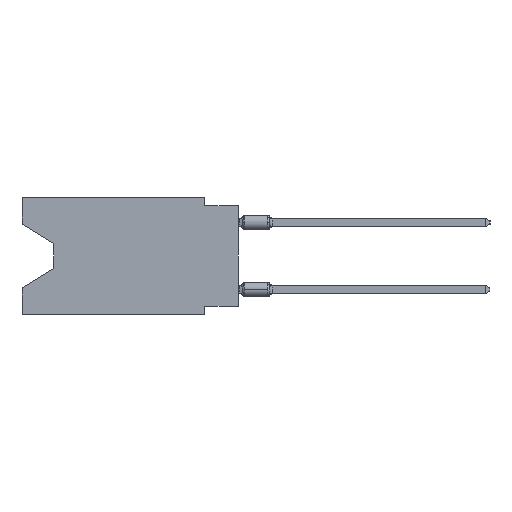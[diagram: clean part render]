
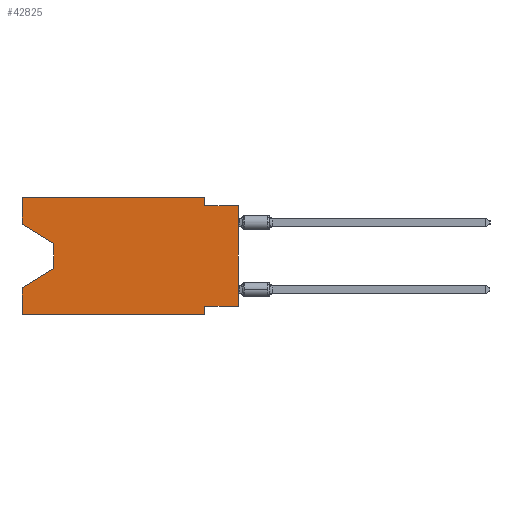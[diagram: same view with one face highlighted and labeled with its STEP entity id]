
A CAD part, left-side view. The second image highlights one B-rep face of the part: STEP entity #42825.
In plain terms, the highlighted planar face has unit normal (-1, 0, 0).
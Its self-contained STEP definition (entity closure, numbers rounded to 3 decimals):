
#413 = VERTEX_POINT ( 'NONE', #1573 ) ;
#453 = EDGE_CURVE ( 'NONE', #9264, #36588, #47007, .T. ) ;
#728 = ORIENTED_EDGE ( 'NONE', *, *, #28625, .T. ) ;
#846 = EDGE_CURVE ( 'NONE', #4577, #4938, #35246, .T. ) ;
#1457 = VERTEX_POINT ( 'NONE', #25924 ) ;
#1476 = VERTEX_POINT ( 'NONE', #22932 ) ;
#1573 = CARTESIAN_POINT ( 'NONE',  ( 0., 2.54, -0.635 ) ) ;
#1760 = EDGE_LOOP ( 'NONE', ( #43189, #728, #45736, #14791, #30633, #1821, #18890, #32439, #21754, #11471, #21118, #30006 ) ) ;
#1821 = ORIENTED_EDGE ( 'NONE', *, *, #45792, .F. ) ;
#2199 = CARTESIAN_POINT ( 'NONE',  ( 0., 0., -0.635 ) ) ;
#2579 = LINE ( 'NONE', #36806, #14096 ) ;
#3229 = LINE ( 'NONE', #21610, #23367 ) ;
#4577 = VERTEX_POINT ( 'NONE', #17387 ) ;
#4938 = VERTEX_POINT ( 'NONE', #22803 ) ;
#5269 = CARTESIAN_POINT ( 'NONE',  ( 0., 0., -0.635 ) ) ;
#7026 = VECTOR ( 'NONE', #13590, 1000. ) ;
#7044 = DIRECTION ( 'NONE',  ( 0., -0.855, -0.519 ) ) ;
#7369 = VERTEX_POINT ( 'NONE', #48970 ) ;
#7563 = VECTOR ( 'NONE', #43129, 1000. ) ;
#9264 = VERTEX_POINT ( 'NONE', #17557 ) ;
#10721 = DIRECTION ( 'NONE',  ( 0., -1., 0. ) ) ;
#11295 = EDGE_CURVE ( 'NONE', #19260, #7369, #37033, .T. ) ;
#11471 = ORIENTED_EDGE ( 'NONE', *, *, #38206, .F. ) ;
#11956 = VECTOR ( 'NONE', #24663, 1000. ) ;
#11966 = EDGE_CURVE ( 'NONE', #16822, #4938, #25248, .T. ) ;
#12874 = DIRECTION ( 'NONE',  ( 0., -1., 0. ) ) ;
#13163 = DIRECTION ( 'NONE',  ( 0., 0.855, -0.519 ) ) ;
#13590 = DIRECTION ( 'NONE',  ( 0., 0., 1. ) ) ;
#13840 = VECTOR ( 'NONE', #38449, 1000. ) ;
#14096 = VECTOR ( 'NONE', #48000, 1000. ) ;
#14159 = DIRECTION ( 'NONE',  ( 0., 0., -1. ) ) ;
#14533 = CARTESIAN_POINT ( 'NONE',  ( 0., 16.383, 0. ) ) ;
#14791 = ORIENTED_EDGE ( 'NONE', *, *, #11966, .F. ) ;
#15324 = CARTESIAN_POINT ( 'NONE',  ( 0., 16.383, 0. ) ) ;
#15622 = CARTESIAN_POINT ( 'NONE',  ( 0., 0., 0. ) ) ;
#15629 = CARTESIAN_POINT ( 'NONE',  ( 0., 16.383, -8.89 ) ) ;
#16266 = EDGE_CURVE ( 'NONE', #37118, #1476, #26870, .T. ) ;
#16571 = LINE ( 'NONE', #31946, #7563 ) ;
#16822 = VERTEX_POINT ( 'NONE', #15629 ) ;
#16841 = LINE ( 'NONE', #2199, #37458 ) ;
#17386 = VECTOR ( 'NONE', #7044, 1000. ) ;
#17387 = CARTESIAN_POINT ( 'NONE',  ( 0., 13.97, -5.385 ) ) ;
#17429 = EDGE_CURVE ( 'NONE', #16822, #1457, #16571, .T. ) ;
#17557 = CARTESIAN_POINT ( 'NONE',  ( 0., 0., -8.255 ) ) ;
#17674 = CARTESIAN_POINT ( 'NONE',  ( 0., 16.383, 0. ) ) ;
#18890 = ORIENTED_EDGE ( 'NONE', *, *, #453, .F. ) ;
#19260 = VERTEX_POINT ( 'NONE', #30118 ) ;
#19389 = VECTOR ( 'NONE', #23039, 1000. ) ;
#21118 = ORIENTED_EDGE ( 'NONE', *, *, #11295, .F. ) ;
#21610 = CARTESIAN_POINT ( 'NONE',  ( 0., 2.54, 0. ) ) ;
#21754 = ORIENTED_EDGE ( 'NONE', *, *, #35468, .F. ) ;
#22803 = CARTESIAN_POINT ( 'NONE',  ( 0., 16.383, -6.852 ) ) ;
#22932 = CARTESIAN_POINT ( 'NONE',  ( 0., 13.97, -3.505 ) ) ;
#23039 = DIRECTION ( 'NONE',  ( 0., 0., 1. ) ) ;
#23367 = VECTOR ( 'NONE', #14159, 1000. ) ;
#23671 = CARTESIAN_POINT ( 'NONE',  ( 0., 2.54, -8.89 ) ) ;
#23829 = CARTESIAN_POINT ( 'NONE',  ( 0., 2.54, -8.255 ) ) ;
#24663 = DIRECTION ( 'NONE',  ( 0., 1., 0. ) ) ;
#25092 = EDGE_CURVE ( 'NONE', #37118, #19260, #38165, .T. ) ;
#25248 = LINE ( 'NONE', #14533, #7026 ) ;
#25924 = CARTESIAN_POINT ( 'NONE',  ( 0., 2.54, -8.89 ) ) ;
#26257 = DIRECTION ( 'NONE',  ( 1., 0., 0. ) ) ;
#26870 = LINE ( 'NONE', #34060, #17386 ) ;
#28625 = EDGE_CURVE ( 'NONE', #1476, #4577, #2579, .T. ) ;
#30006 = ORIENTED_EDGE ( 'NONE', *, *, #25092, .F. ) ;
#30010 = VERTEX_POINT ( 'NONE', #5269 ) ;
#30118 = CARTESIAN_POINT ( 'NONE',  ( 0., 16.383, 0. ) ) ;
#30517 = LINE ( 'NONE', #15622, #13840 ) ;
#30633 = ORIENTED_EDGE ( 'NONE', *, *, #17429, .T. ) ;
#31340 = LINE ( 'NONE', #23671, #33969 ) ;
#31946 = CARTESIAN_POINT ( 'NONE',  ( 0., 16.383, -8.89 ) ) ;
#32439 = ORIENTED_EDGE ( 'NONE', *, *, #37629, .T. ) ;
#33184 = VECTOR ( 'NONE', #10721, 1000. ) ;
#33969 = VECTOR ( 'NONE', #34079, 1000. ) ;
#34060 = CARTESIAN_POINT ( 'NONE',  ( 0., 16.383, -2.038 ) ) ;
#34079 = DIRECTION ( 'NONE',  ( 0., 0., -1. ) ) ;
#35246 = LINE ( 'NONE', #47185, #44467 ) ;
#35468 = EDGE_CURVE ( 'NONE', #413, #30010, #16841, .T. ) ;
#36522 = FACE_OUTER_BOUND ( 'NONE', #1760, .T. ) ;
#36588 = VERTEX_POINT ( 'NONE', #23829 ) ;
#36806 = CARTESIAN_POINT ( 'NONE',  ( 0., 13.97, -3.505 ) ) ;
#37033 = LINE ( 'NONE', #17674, #33184 ) ;
#37036 = AXIS2_PLACEMENT_3D ( 'NONE', #45361, #26257, #38154 ) ;
#37118 = VERTEX_POINT ( 'NONE', #40356 ) ;
#37458 = VECTOR ( 'NONE', #12874, 1000. ) ;
#37629 = EDGE_CURVE ( 'NONE', #9264, #30010, #30517, .T. ) ;
#38154 = DIRECTION ( 'NONE',  ( 0., 0., -1. ) ) ;
#38165 = LINE ( 'NONE', #15324, #19389 ) ;
#38206 = EDGE_CURVE ( 'NONE', #7369, #413, #3229, .T. ) ;
#38449 = DIRECTION ( 'NONE',  ( 0., 0., 1. ) ) ;
#40016 = CARTESIAN_POINT ( 'NONE',  ( 0., 0., -8.255 ) ) ;
#40356 = CARTESIAN_POINT ( 'NONE',  ( 0., 16.383, -2.038 ) ) ;
#42825 = ADVANCED_FACE ( 'NONE', ( #36522 ), #47942, .F. ) ;
#43129 = DIRECTION ( 'NONE',  ( 0., -1., 0. ) ) ;
#43189 = ORIENTED_EDGE ( 'NONE', *, *, #16266, .T. ) ;
#44467 = VECTOR ( 'NONE', #13163, 1000. ) ;
#45361 = CARTESIAN_POINT ( 'NONE',  ( 0., 16.383, 0. ) ) ;
#45736 = ORIENTED_EDGE ( 'NONE', *, *, #846, .T. ) ;
#45792 = EDGE_CURVE ( 'NONE', #36588, #1457, #31340, .T. ) ;
#47007 = LINE ( 'NONE', #40016, #11956 ) ;
#47185 = CARTESIAN_POINT ( 'NONE',  ( 0., 13.97, -5.385 ) ) ;
#47942 = PLANE ( 'NONE',  #37036 ) ;
#48000 = DIRECTION ( 'NONE',  ( 0., 0., -1. ) ) ;
#48970 = CARTESIAN_POINT ( 'NONE',  ( 0., 2.54, 0. ) ) ;
